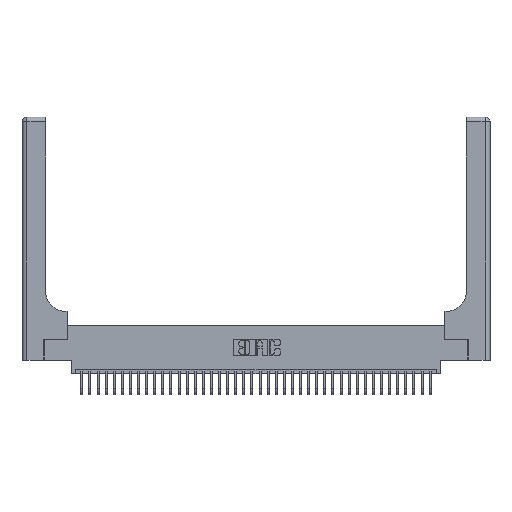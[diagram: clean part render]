
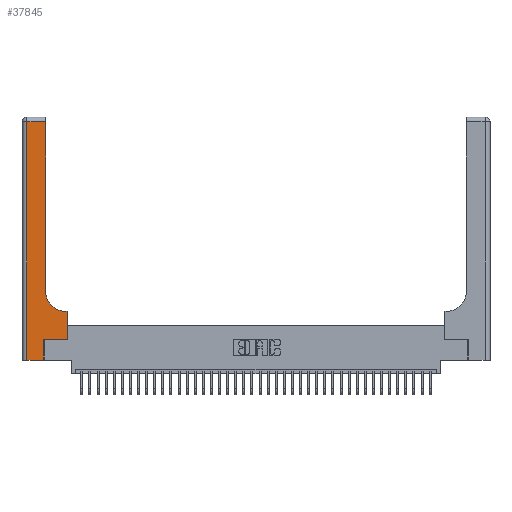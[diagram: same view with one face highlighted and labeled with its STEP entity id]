
A CAD part, top view. The second image highlights one B-rep face of the part: STEP entity #37845.
In plain terms, the highlighted planar face has unit normal (0, 0, 1).
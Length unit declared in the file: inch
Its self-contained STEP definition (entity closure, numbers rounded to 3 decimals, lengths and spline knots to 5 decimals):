
#521 = CARTESIAN_POINT ( 'NONE',  ( 0.269, 0., 0.37 ) ) ;
#1445 = EDGE_CURVE ( 'NONE', #39924, #25444, #32171, .T. ) ;
#1526 = FACE_OUTER_BOUND ( 'NONE', #26273, .T. ) ;
#3120 = VERTEX_POINT ( 'NONE', #39757 ) ;
#3529 = CARTESIAN_POINT ( 'NONE',  ( 0.2915, 2.94, 0.37 ) ) ;
#4792 = DIRECTION ( 'NONE',  ( 0., 0., -1. ) ) ;
#4912 = VECTOR ( 'NONE', #33650, 39.37008 ) ;
#5587 = EDGE_CURVE ( 'NONE', #22324, #39924, #21748, .T. ) ;
#7154 = CARTESIAN_POINT ( 'NONE',  ( 0., 0., 0.37 ) ) ;
#8119 = CARTESIAN_POINT ( 'NONE',  ( 0.269, 0.25, 0.37 ) ) ;
#8408 = EDGE_CURVE ( 'NONE', #3120, #33860, #28326, .T. ) ;
#8647 = CARTESIAN_POINT ( 'NONE',  ( 0.06, 2.94, 0.37 ) ) ;
#9514 = EDGE_CURVE ( 'NONE', #15166, #24838, #21713, .T. ) ;
#9589 = DIRECTION ( 'NONE',  ( 0., 1., 0. ) ) ;
#9745 = EDGE_CURVE ( 'NONE', #24173, #22324, #40621, .T. ) ;
#10478 = EDGE_CURVE ( 'NONE', #25444, #3120, #36704, .T. ) ;
#11303 = DIRECTION ( 'NONE',  ( 1., 0., 0. ) ) ;
#11844 = CARTESIAN_POINT ( 'NONE',  ( 0., 2.94, 0.37 ) ) ;
#12418 = LINE ( 'NONE', #30481, #4912 ) ;
#12675 = AXIS2_PLACEMENT_3D ( 'NONE', #35398, #19530, #33178 ) ;
#14713 = DIRECTION ( 'NONE',  ( -1., 0., 0. ) ) ;
#15044 = DIRECTION ( 'NONE',  ( -1., 0., 0. ) ) ;
#15166 = VERTEX_POINT ( 'NONE', #27032 ) ;
#15324 = CARTESIAN_POINT ( 'NONE',  ( 0.269, 0., 0.37 ) ) ;
#15690 = VERTEX_POINT ( 'NONE', #20190 ) ;
#15733 = ORIENTED_EDGE ( 'NONE', *, *, #9745, .T. ) ;
#15858 = VECTOR ( 'NONE', #11303, 39.37008 ) ;
#16309 = DIRECTION ( 'NONE',  ( 1., 0., 0. ) ) ;
#19137 = ORIENTED_EDGE ( 'NONE', *, *, #5587, .T. ) ;
#19530 = DIRECTION ( 'NONE',  ( 0., 0., -1. ) ) ;
#20190 = CARTESIAN_POINT ( 'NONE',  ( 0.5585, 0.6, 0.37 ) ) ;
#20464 = ORIENTED_EDGE ( 'NONE', *, *, #10478, .T. ) ;
#21081 = PLANE ( 'NONE',  #40723 ) ;
#21240 = VECTOR ( 'NONE', #16309, 39.37008 ) ;
#21713 = LINE ( 'NONE', #8119, #21240 ) ;
#21748 = LINE ( 'NONE', #29855, #28241 ) ;
#22324 = VERTEX_POINT ( 'NONE', #22870 ) ;
#22870 = CARTESIAN_POINT ( 'NONE',  ( 0.2915, 0.85, 0.37 ) ) ;
#23164 = VECTOR ( 'NONE', #15044, 39.37008 ) ;
#23549 = ORIENTED_EDGE ( 'NONE', *, *, #30971, .T. ) ;
#24173 = VERTEX_POINT ( 'NONE', #35811 ) ;
#24541 = CARTESIAN_POINT ( 'NONE',  ( 0.5585, 0.25, 0.37 ) ) ;
#24646 = VECTOR ( 'NONE', #32342, 39.37008 ) ;
#24838 = VERTEX_POINT ( 'NONE', #24541 ) ;
#25444 = VERTEX_POINT ( 'NONE', #8647 ) ;
#25978 = ORIENTED_EDGE ( 'NONE', *, *, #8408, .T. ) ;
#26273 = EDGE_LOOP ( 'NONE', ( #19137, #31399, #20464, #25978, #23549, #35624, #31512, #35382, #15733 ) ) ;
#26896 = DIRECTION ( 'NONE',  ( 0., 1., 0. ) ) ;
#27032 = CARTESIAN_POINT ( 'NONE',  ( 0.269, 0.25, 0.37 ) ) ;
#28241 = VECTOR ( 'NONE', #26896, 39.37008 ) ;
#28258 = VECTOR ( 'NONE', #38531, 39.37008 ) ;
#28326 = LINE ( 'NONE', #7154, #15858 ) ;
#29510 = CARTESIAN_POINT ( 'NONE',  ( 0.06, 3., 0.37 ) ) ;
#29855 = CARTESIAN_POINT ( 'NONE',  ( 0.2915, 3., 0.37 ) ) ;
#30438 = CARTESIAN_POINT ( 'NONE',  ( 0., 3., 0.37 ) ) ;
#30481 = CARTESIAN_POINT ( 'NONE',  ( 0.2915, 0.6, 0.37 ) ) ;
#30971 = EDGE_CURVE ( 'NONE', #33860, #15166, #33949, .T. ) ;
#31399 = ORIENTED_EDGE ( 'NONE', *, *, #1445, .T. ) ;
#31512 = ORIENTED_EDGE ( 'NONE', *, *, #35149, .T. ) ;
#32171 = LINE ( 'NONE', #11844, #23164 ) ;
#32342 = DIRECTION ( 'NONE',  ( 0., 1., 0. ) ) ;
#32662 = EDGE_CURVE ( 'NONE', #15690, #24173, #12418, .T. ) ;
#33178 = DIRECTION ( 'NONE',  ( 1., 0., 0. ) ) ;
#33650 = DIRECTION ( 'NONE',  ( -1., 0., 0. ) ) ;
#33860 = VERTEX_POINT ( 'NONE', #521 ) ;
#33949 = LINE ( 'NONE', #15324, #38943 ) ;
#35149 = EDGE_CURVE ( 'NONE', #24838, #15690, #39569, .T. ) ;
#35382 = ORIENTED_EDGE ( 'NONE', *, *, #32662, .T. ) ;
#35398 = CARTESIAN_POINT ( 'NONE',  ( 0.5415, 0.85, 0.37 ) ) ;
#35624 = ORIENTED_EDGE ( 'NONE', *, *, #9514, .T. ) ;
#35811 = CARTESIAN_POINT ( 'NONE',  ( 0.5415, 0.6, 0.37 ) ) ;
#36704 = LINE ( 'NONE', #29510, #28258 ) ;
#37845 = ADVANCED_FACE ( 'NONE', ( #1526 ), #21081, .F. ) ;
#38531 = DIRECTION ( 'NONE',  ( 0., -1., 0. ) ) ;
#38590 = CARTESIAN_POINT ( 'NONE',  ( 0.5585, 0.25, 0.37 ) ) ;
#38943 = VECTOR ( 'NONE', #9589, 39.37008 ) ;
#39569 = LINE ( 'NONE', #38590, #24646 ) ;
#39757 = CARTESIAN_POINT ( 'NONE',  ( 0.06, 0., 0.37 ) ) ;
#39924 = VERTEX_POINT ( 'NONE', #3529 ) ;
#40621 = CIRCLE ( 'NONE', #12675, 0.25 ) ;
#40723 = AXIS2_PLACEMENT_3D ( 'NONE', #30438, #4792, #14713 ) ;
